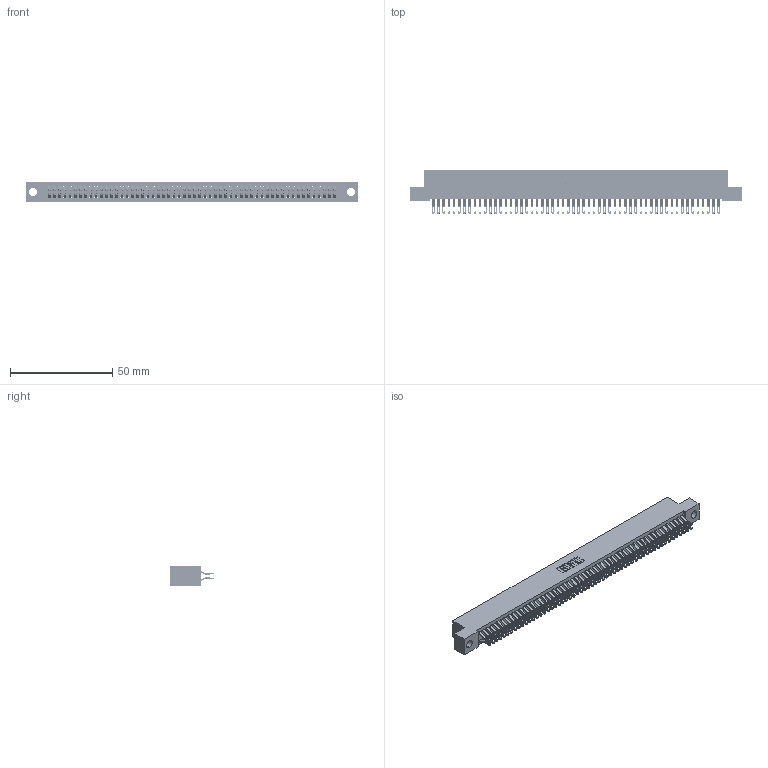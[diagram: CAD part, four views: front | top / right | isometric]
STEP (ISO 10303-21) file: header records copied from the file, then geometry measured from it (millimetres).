
FILE_DESCRIPTION (( 'STEP AP203' ), '1' );
FILE_NAME ('392-112-555-204.STEP', '2018-08-18T22:42:17', ( '' ), ( '' ), 'SwSTEP 2.0', 'SolidWorks 2016', '' );
FILE_SCHEMA (( 'CONFIG_CONTROL_DESIGN' ));
Length unit declared in the file: inch
Products named in the file (3): 342 Part_.156 TH; 345-292-001_555 Tail; 392-112-555-204
Assembly tree (113 placements, depth 2):
  392-112-555-204
    342 Part_.156 TH
    345-292-001_555 Tail  x112
Bounding box: 162.56 x 21.47 x 9.4 mm (x, y, z)
Volume: 14896.5 mm3; surface area: 25500.6 mm2
Topology: 113 solids, 113 shells, 6606 faces, 20795 edges, 13862 vertices
Faces by surface type: plane 3874, cylinder 2732
Entity records: 34413 total; most frequent: CARTESIAN_POINT 5720, ORIENTED_EDGE 5626, DIRECTION 4833, EDGE_CURVE 2813, VECTOR 2665, LINE 2665, VERTEX_POINT 1874, AXIS2_PLACEMENT_3D 1084
